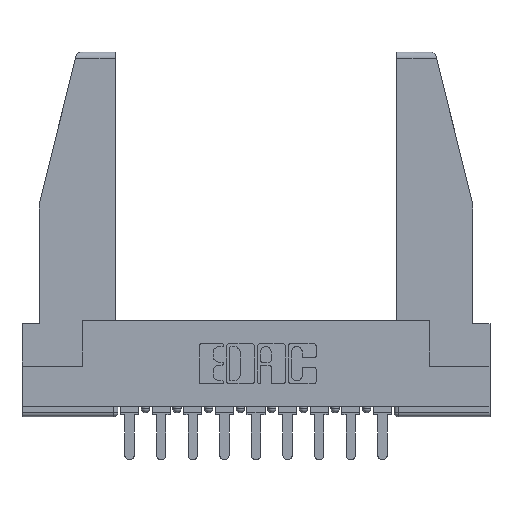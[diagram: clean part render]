
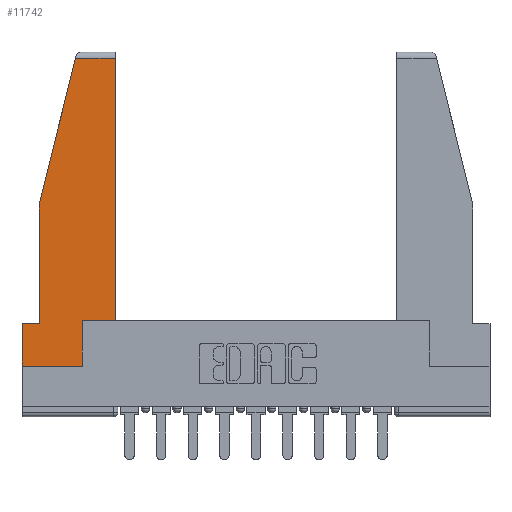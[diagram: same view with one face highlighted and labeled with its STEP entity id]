
A CAD part, top view. The second image highlights one B-rep face of the part: STEP entity #11742.
In plain terms, the highlighted planar face has unit normal (0, 0, 1).
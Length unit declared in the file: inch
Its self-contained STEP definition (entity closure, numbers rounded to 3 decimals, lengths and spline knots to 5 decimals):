
#315 = ORIENTED_EDGE ( 'NONE', *, *, #11302, .T. ) ;
#492 = CARTESIAN_POINT ( 'NONE',  ( 0.297, 0., 0. ) ) ;
#562 = DIRECTION ( 'NONE',  ( 1., 0., 0. ) ) ;
#719 = CARTESIAN_POINT ( 'NONE',  ( 0., 0., 0. ) ) ;
#852 = CARTESIAN_POINT ( 'NONE',  ( 0., 1.52, 0. ) ) ;
#854 = FACE_OUTER_BOUND ( 'NONE', #14910, .T. ) ;
#913 = DIRECTION ( 'NONE',  ( 0., -1., 0. ) ) ;
#1039 = VECTOR ( 'NONE', #9265, 39.37008 ) ;
#1298 = ORIENTED_EDGE ( 'NONE', *, *, #2257, .T. ) ;
#1325 = CARTESIAN_POINT ( 'NONE',  ( 0.461, 0.223, 0. ) ) ;
#1666 = DIRECTION ( 'NONE',  ( 0., -1., 0. ) ) ;
#1778 = ORIENTED_EDGE ( 'NONE', *, *, #4148, .T. ) ;
#2257 = EDGE_CURVE ( 'NONE', #2352, #6397, #10627, .T. ) ;
#2352 = VERTEX_POINT ( 'NONE', #2816 ) ;
#2761 = VECTOR ( 'NONE', #11679, 39.37008 ) ;
#2799 = PLANE ( 'NONE',  #6726 ) ;
#2816 = CARTESIAN_POINT ( 'NONE',  ( 0.2636, 1.52, 0. ) ) ;
#3275 = ORIENTED_EDGE ( 'NONE', *, *, #12049, .T. ) ;
#3528 = VECTOR ( 'NONE', #4552, 39.37008 ) ;
#4008 = DIRECTION ( 'NONE',  ( 0., 1., 0. ) ) ;
#4067 = LINE ( 'NONE', #1325, #1039 ) ;
#4148 = EDGE_CURVE ( 'NONE', #8619, #9471, #13084, .T. ) ;
#4304 = CARTESIAN_POINT ( 'NONE',  ( 0.271, 1.55, 0. ) ) ;
#4454 = DIRECTION ( 'NONE',  ( 1., 0., 0. ) ) ;
#4552 = DIRECTION ( 'NONE',  ( -0.239, -0.971, 0. ) ) ;
#5118 = CARTESIAN_POINT ( 'NONE',  ( 0.297, 0., 0. ) ) ;
#5562 = LINE ( 'NONE', #719, #14463 ) ;
#5719 = CARTESIAN_POINT ( 'NONE',  ( 0., 0., 0. ) ) ;
#5758 = VECTOR ( 'NONE', #11712, 39.37008 ) ;
#6239 = VERTEX_POINT ( 'NONE', #5719 ) ;
#6264 = LINE ( 'NONE', #7782, #14808 ) ;
#6397 = VERTEX_POINT ( 'NONE', #14050 ) ;
#6415 = CARTESIAN_POINT ( 'NONE',  ( 0.086, 0.21, 0. ) ) ;
#6726 = AXIS2_PLACEMENT_3D ( 'NONE', #12000, #10910, #562 ) ;
#7051 = ORIENTED_EDGE ( 'NONE', *, *, #9329, .T. ) ;
#7165 = LINE ( 'NONE', #13387, #13362 ) ;
#7425 = CARTESIAN_POINT ( 'NONE',  ( 0.461, 0.223, 0. ) ) ;
#7782 = CARTESIAN_POINT ( 'NONE',  ( 0., 0.21, 0. ) ) ;
#7982 = LINE ( 'NONE', #5118, #10383 ) ;
#8151 = CARTESIAN_POINT ( 'NONE',  ( 0.297, 0.223, 0. ) ) ;
#8194 = CARTESIAN_POINT ( 'NONE',  ( 0., 0.21, 0. ) ) ;
#8221 = EDGE_CURVE ( 'NONE', #12654, #9389, #11753, .T. ) ;
#8619 = VERTEX_POINT ( 'NONE', #6415 ) ;
#9265 = DIRECTION ( 'NONE',  ( 0., 1., 0. ) ) ;
#9329 = EDGE_CURVE ( 'NONE', #6397, #8619, #7165, .T. ) ;
#9389 = VERTEX_POINT ( 'NONE', #7425 ) ;
#9471 = VERTEX_POINT ( 'NONE', #10101 ) ;
#9520 = EDGE_CURVE ( 'NONE', #9471, #6239, #6264, .T. ) ;
#9570 = CARTESIAN_POINT ( 'NONE',  ( 0.297, 0.223, 0. ) ) ;
#10101 = CARTESIAN_POINT ( 'NONE',  ( 0., 0.21, 0. ) ) ;
#10383 = VECTOR ( 'NONE', #4008, 39.37008 ) ;
#10627 = LINE ( 'NONE', #4304, #3528 ) ;
#10910 = DIRECTION ( 'NONE',  ( 0., 0., 1. ) ) ;
#11011 = CARTESIAN_POINT ( 'NONE',  ( 0.461, 1.52, 0. ) ) ;
#11064 = ORIENTED_EDGE ( 'NONE', *, *, #14267, .T. ) ;
#11085 = LINE ( 'NONE', #852, #13602 ) ;
#11302 = EDGE_CURVE ( 'NONE', #6239, #14648, #5562, .T. ) ;
#11679 = DIRECTION ( 'NONE',  ( -1., 0., 0. ) ) ;
#11712 = DIRECTION ( 'NONE',  ( 1., 0., 0. ) ) ;
#11742 = ADVANCED_FACE ( 'NONE', ( #854 ), #2799, .T. ) ;
#11753 = LINE ( 'NONE', #9570, #5758 ) ;
#12000 = CARTESIAN_POINT ( 'NONE',  ( 0., 0., 0. ) ) ;
#12049 = EDGE_CURVE ( 'NONE', #9389, #14093, #4067, .T. ) ;
#12311 = ORIENTED_EDGE ( 'NONE', *, *, #8221, .T. ) ;
#12502 = DIRECTION ( 'NONE',  ( -1., 0., 0. ) ) ;
#12654 = VERTEX_POINT ( 'NONE', #8151 ) ;
#12998 = ORIENTED_EDGE ( 'NONE', *, *, #9520, .T. ) ;
#13084 = LINE ( 'NONE', #8194, #2761 ) ;
#13263 = ORIENTED_EDGE ( 'NONE', *, *, #13422, .T. ) ;
#13362 = VECTOR ( 'NONE', #1666, 39.37008 ) ;
#13387 = CARTESIAN_POINT ( 'NONE',  ( 0.086, 0.8, 0. ) ) ;
#13422 = EDGE_CURVE ( 'NONE', #14648, #12654, #7982, .T. ) ;
#13602 = VECTOR ( 'NONE', #12502, 39.37008 ) ;
#14050 = CARTESIAN_POINT ( 'NONE',  ( 0.086, 0.8, 0. ) ) ;
#14093 = VERTEX_POINT ( 'NONE', #11011 ) ;
#14267 = EDGE_CURVE ( 'NONE', #14093, #2352, #11085, .T. ) ;
#14463 = VECTOR ( 'NONE', #4454, 39.37008 ) ;
#14648 = VERTEX_POINT ( 'NONE', #492 ) ;
#14808 = VECTOR ( 'NONE', #913, 39.37008 ) ;
#14910 = EDGE_LOOP ( 'NONE', ( #3275, #11064, #1298, #7051, #1778, #12998, #315, #13263, #12311 ) ) ;
